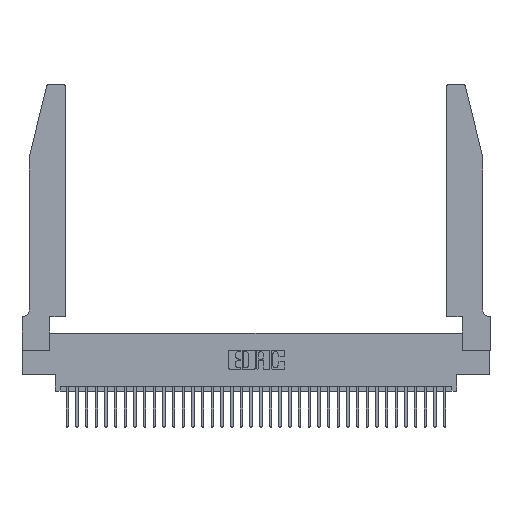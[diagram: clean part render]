
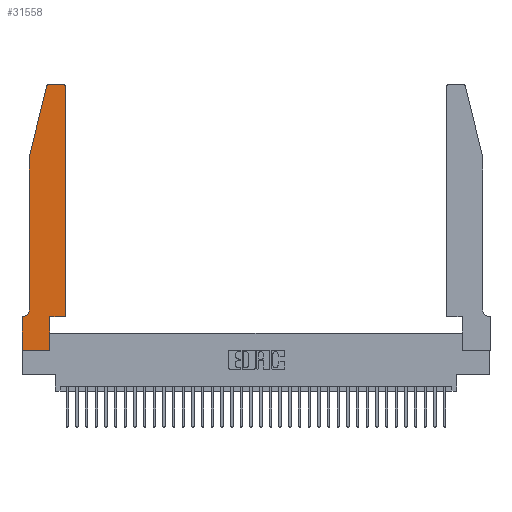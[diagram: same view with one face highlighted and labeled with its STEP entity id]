
A CAD part, top view. The second image highlights one B-rep face of the part: STEP entity #31558.
In plain terms, the highlighted planar face has unit normal (0, 0, 1).
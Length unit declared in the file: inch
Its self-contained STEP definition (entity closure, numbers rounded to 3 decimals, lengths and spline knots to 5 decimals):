
#194 = CARTESIAN_POINT ( 'NONE',  ( 0.2605, 2.75, 0.37 ) ) ;
#349 = EDGE_CURVE ( 'NONE', #7827, #1847, #3192, .T. ) ;
#558 = CARTESIAN_POINT ( 'NONE',  ( 0.4205, 2.75, 0.37 ) ) ;
#727 = EDGE_CURVE ( 'NONE', #35272, #1293, #13643, .T. ) ;
#1282 = CARTESIAN_POINT ( 'NONE',  ( 0.4205, 2.72, 0.37 ) ) ;
#1293 = VERTEX_POINT ( 'NONE', #11244 ) ;
#1847 = VERTEX_POINT ( 'NONE', #33084 ) ;
#2599 = CARTESIAN_POINT ( 'NONE',  ( 0.0755, 0.42, 0.37 ) ) ;
#3192 = LINE ( 'NONE', #6505, #26534 ) ;
#3485 = CARTESIAN_POINT ( 'NONE',  ( 0.4505, 0.35, 0.37 ) ) ;
#3593 = CARTESIAN_POINT ( 'NONE',  ( 0.0055, 0.42, 0.37 ) ) ;
#3764 = DIRECTION ( 'NONE',  ( 0., -1., 0. ) ) ;
#4262 = DIRECTION ( 'NONE',  ( -1., 0., 0. ) ) ;
#5376 = VECTOR ( 'NONE', #25565, 39.37008 ) ;
#5449 = VERTEX_POINT ( 'NONE', #22663 ) ;
#5545 = CARTESIAN_POINT ( 'NONE',  ( 0.2865, 0.35, 0.37 ) ) ;
#6414 = DIRECTION ( 'NONE',  ( 1., 0., 0. ) ) ;
#6505 = CARTESIAN_POINT ( 'NONE',  ( 0., 0., 0.37 ) ) ;
#6681 = ORIENTED_EDGE ( 'NONE', *, *, #13092, .T. ) ;
#7019 = EDGE_CURVE ( 'NONE', #32233, #9240, #11593, .T. ) ;
#7063 = DIRECTION ( 'NONE',  ( 1., 0., 0. ) ) ;
#7517 = FACE_OUTER_BOUND ( 'NONE', #9858, .T. ) ;
#7609 = ORIENTED_EDGE ( 'NONE', *, *, #35961, .T. ) ;
#7827 = VERTEX_POINT ( 'NONE', #34136 ) ;
#9240 = VERTEX_POINT ( 'NONE', #28035 ) ;
#9483 = AXIS2_PLACEMENT_3D ( 'NONE', #1282, #20833, #7063 ) ;
#9858 = EDGE_LOOP ( 'NONE', ( #24579, #34644, #22893, #31028, #28174, #14202, #17123, #12031, #7609, #19201, #6681, #23134 ) ) ;
#10164 = VECTOR ( 'NONE', #19861, 39.37008 ) ;
#10455 = DIRECTION ( 'NONE',  ( 0., 1., 0. ) ) ;
#11244 = CARTESIAN_POINT ( 'NONE',  ( 0.0755, 2., 0.37 ) ) ;
#11503 = CARTESIAN_POINT ( 'NONE',  ( 0., 0.35, 0.37 ) ) ;
#11593 = LINE ( 'NONE', #194, #29115 ) ;
#12031 = ORIENTED_EDGE ( 'NONE', *, *, #32986, .T. ) ;
#12198 = LINE ( 'NONE', #12205, #13123 ) ;
#12205 = CARTESIAN_POINT ( 'NONE',  ( 0., 0., 0.37 ) ) ;
#12365 = LINE ( 'NONE', #16827, #5376 ) ;
#12510 = VECTOR ( 'NONE', #14279, 39.37008 ) ;
#12933 = LINE ( 'NONE', #27282, #30597 ) ;
#13092 = EDGE_CURVE ( 'NONE', #29105, #5449, #12933, .T. ) ;
#13123 = VECTOR ( 'NONE', #6414, 39.37008 ) ;
#13643 = LINE ( 'NONE', #23633, #28564 ) ;
#14202 = ORIENTED_EDGE ( 'NONE', *, *, #17690, .T. ) ;
#14279 = DIRECTION ( 'NONE',  ( 0., 1., 0. ) ) ;
#15644 = VERTEX_POINT ( 'NONE', #2599 ) ;
#15665 = AXIS2_PLACEMENT_3D ( 'NONE', #3593, #20590, #26267 ) ;
#16757 = CARTESIAN_POINT ( 'NONE',  ( 0.284, 2.72, 0.37 ) ) ;
#16827 = CARTESIAN_POINT ( 'NONE',  ( 0.4505, 0.35, 0.37 ) ) ;
#17026 = DIRECTION ( 'NONE',  ( 1., 0., 0. ) ) ;
#17123 = ORIENTED_EDGE ( 'NONE', *, *, #349, .T. ) ;
#17690 = EDGE_CURVE ( 'NONE', #19146, #7827, #25595, .T. ) ;
#18493 = LINE ( 'NONE', #30933, #10164 ) ;
#19146 = VERTEX_POINT ( 'NONE', #25547 ) ;
#19201 = ORIENTED_EDGE ( 'NONE', *, *, #30836, .T. ) ;
#19296 = CARTESIAN_POINT ( 'NONE',  ( 0.2865, 0.35, 0.37 ) ) ;
#19605 = DIRECTION ( 'NONE',  ( 0., 0., 1. ) ) ;
#19749 = DIRECTION ( 'NONE',  ( 0., 0., 1. ) ) ;
#19861 = DIRECTION ( 'NONE',  ( 0., -1., 0. ) ) ;
#20590 = DIRECTION ( 'NONE',  ( 0., 0., -1. ) ) ;
#20833 = DIRECTION ( 'NONE',  ( 0., 0., 1. ) ) ;
#20868 = LINE ( 'NONE', #5545, #12510 ) ;
#21624 = VECTOR ( 'NONE', #32314, 39.37008 ) ;
#22456 = EDGE_CURVE ( 'NONE', #5449, #32233, #29108, .T. ) ;
#22663 = CARTESIAN_POINT ( 'NONE',  ( 0.4505, 2.72, 0.37 ) ) ;
#22893 = ORIENTED_EDGE ( 'NONE', *, *, #727, .T. ) ;
#23134 = ORIENTED_EDGE ( 'NONE', *, *, #22456, .T. ) ;
#23633 = CARTESIAN_POINT ( 'NONE',  ( 0.0755, 2., 0.37 ) ) ;
#23833 = VERTEX_POINT ( 'NONE', #35121 ) ;
#24579 = ORIENTED_EDGE ( 'NONE', *, *, #7019, .T. ) ;
#25547 = CARTESIAN_POINT ( 'NONE',  ( 0.0055, 0.35, 0.37 ) ) ;
#25565 = DIRECTION ( 'NONE',  ( 1., 0., 0. ) ) ;
#25595 = LINE ( 'NONE', #29223, #21624 ) ;
#26032 = AXIS2_PLACEMENT_3D ( 'NONE', #16757, #19605, #27971 ) ;
#26130 = EDGE_CURVE ( 'NONE', #15644, #19146, #32342, .T. ) ;
#26267 = DIRECTION ( 'NONE',  ( -1., 0., 0. ) ) ;
#26534 = VECTOR ( 'NONE', #3764, 39.37008 ) ;
#27282 = CARTESIAN_POINT ( 'NONE',  ( 0.4505, 0.35, 0.37 ) ) ;
#27744 = CARTESIAN_POINT ( 'NONE',  ( 0.25487, 2.72718, 0.37 ) ) ;
#27971 = DIRECTION ( 'NONE',  ( 1., 0., 0. ) ) ;
#28035 = CARTESIAN_POINT ( 'NONE',  ( 0.284, 2.75, 0.37 ) ) ;
#28174 = ORIENTED_EDGE ( 'NONE', *, *, #26130, .T. ) ;
#28564 = VECTOR ( 'NONE', #32427, 39.37008 ) ;
#29105 = VERTEX_POINT ( 'NONE', #3485 ) ;
#29108 = CIRCLE ( 'NONE', #9483, 0.03 ) ;
#29115 = VECTOR ( 'NONE', #4262, 39.37008 ) ;
#29223 = CARTESIAN_POINT ( 'NONE',  ( 0.0755, 0.35, 0.37 ) ) ;
#30597 = VECTOR ( 'NONE', #10455, 39.37008 ) ;
#30836 = EDGE_CURVE ( 'NONE', #34590, #29105, #12365, .T. ) ;
#30933 = CARTESIAN_POINT ( 'NONE',  ( 0.0755, 2., 0.37 ) ) ;
#31028 = ORIENTED_EDGE ( 'NONE', *, *, #31543, .T. ) ;
#31543 = EDGE_CURVE ( 'NONE', #1293, #15644, #18493, .T. ) ;
#31558 = ADVANCED_FACE ( 'NONE', ( #7517 ), #33890, .T. ) ;
#31882 = EDGE_CURVE ( 'NONE', #9240, #35272, #36195, .T. ) ;
#32233 = VERTEX_POINT ( 'NONE', #558 ) ;
#32314 = DIRECTION ( 'NONE',  ( -1., 0., 0. ) ) ;
#32342 = CIRCLE ( 'NONE', #15665, 0.07 ) ;
#32427 = DIRECTION ( 'NONE',  ( -0.239, -0.971, 0. ) ) ;
#32986 = EDGE_CURVE ( 'NONE', #1847, #23833, #12198, .T. ) ;
#33084 = CARTESIAN_POINT ( 'NONE',  ( 0., 0., 0.37 ) ) ;
#33842 = AXIS2_PLACEMENT_3D ( 'NONE', #11503, #19749, #17026 ) ;
#33890 = PLANE ( 'NONE',  #33842 ) ;
#34136 = CARTESIAN_POINT ( 'NONE',  ( 0., 0.35, 0.37 ) ) ;
#34590 = VERTEX_POINT ( 'NONE', #19296 ) ;
#34644 = ORIENTED_EDGE ( 'NONE', *, *, #31882, .T. ) ;
#35121 = CARTESIAN_POINT ( 'NONE',  ( 0.2865, 0., 0.37 ) ) ;
#35272 = VERTEX_POINT ( 'NONE', #27744 ) ;
#35961 = EDGE_CURVE ( 'NONE', #23833, #34590, #20868, .T. ) ;
#36195 = CIRCLE ( 'NONE', #26032, 0.03 ) ;
